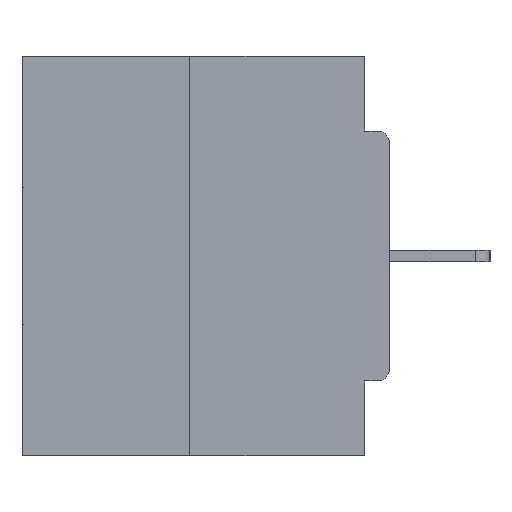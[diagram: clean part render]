
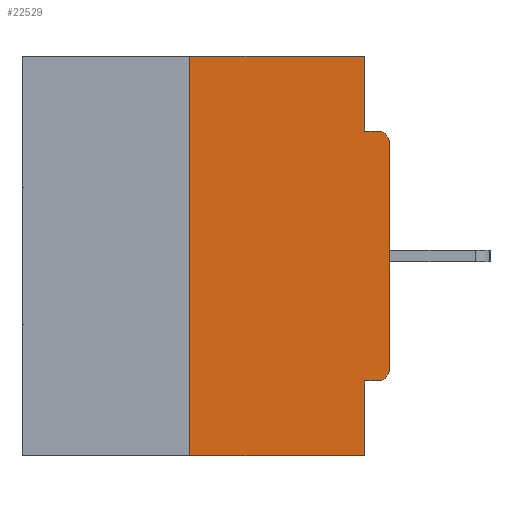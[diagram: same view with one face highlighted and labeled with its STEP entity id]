
A CAD part, left-side view. The second image highlights one B-rep face of the part: STEP entity #22529.
In plain terms, the highlighted planar face has unit normal (-1, 0, 0).
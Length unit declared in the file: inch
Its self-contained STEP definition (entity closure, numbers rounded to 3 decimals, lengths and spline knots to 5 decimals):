
#791 = VERTEX_POINT ( 'NONE', #9020 ) ;
#836 = ORIENTED_EDGE ( 'NONE', *, *, #27586, .F. ) ;
#877 = ORIENTED_EDGE ( 'NONE', *, *, #22318, .F. ) ;
#1056 = DIRECTION ( 'NONE',  ( 0., -1., 0. ) ) ;
#1707 = VECTOR ( 'NONE', #7254, 39.37008 ) ;
#1760 = CARTESIAN_POINT ( 'NONE',  ( 0., 0.25, 0. ) ) ;
#1771 = CIRCLE ( 'NONE', #20552, 0.015 ) ;
#2193 = CARTESIAN_POINT ( 'NONE',  ( 0., 0.46, 0. ) ) ;
#2301 = CARTESIAN_POINT ( 'NONE',  ( 0., 0., -0.0935 ) ) ;
#2384 = DIRECTION ( 'NONE',  ( 0., 0., -1. ) ) ;
#2485 = ORIENTED_EDGE ( 'NONE', *, *, #24553, .T. ) ;
#3978 = CARTESIAN_POINT ( 'NONE',  ( 0., 0.031, -0.4065 ) ) ;
#4126 = LINE ( 'NONE', #1760, #17793 ) ;
#4896 = LINE ( 'NONE', #2193, #1707 ) ;
#6271 = LINE ( 'NONE', #9110, #28137 ) ;
#6667 = DIRECTION ( 'NONE',  ( -1., 0., 0. ) ) ;
#6724 = ORIENTED_EDGE ( 'NONE', *, *, #23701, .F. ) ;
#7254 = DIRECTION ( 'NONE',  ( 0., -1., 0. ) ) ;
#7562 = ORIENTED_EDGE ( 'NONE', *, *, #19030, .T. ) ;
#7564 = DIRECTION ( 'NONE',  ( 0., 0., -1. ) ) ;
#7606 = CARTESIAN_POINT ( 'NONE',  ( 0., 0., -0.1085 ) ) ;
#7730 = EDGE_CURVE ( 'NONE', #12443, #24600, #21650, .T. ) ;
#8236 = DIRECTION ( 'NONE',  ( 1., 0., 0. ) ) ;
#8648 = VERTEX_POINT ( 'NONE', #8951 ) ;
#8951 = CARTESIAN_POINT ( 'NONE',  ( 0., 0.25, -0.5 ) ) ;
#9020 = CARTESIAN_POINT ( 'NONE',  ( 0., 0.25, 0. ) ) ;
#9110 = CARTESIAN_POINT ( 'NONE',  ( 0., 0.46, -0.5 ) ) ;
#9369 = VERTEX_POINT ( 'NONE', #7606 ) ;
#9497 = DIRECTION ( 'NONE',  ( 0., 1., 0. ) ) ;
#10043 = DIRECTION ( 'NONE',  ( 0., -1., 0. ) ) ;
#10325 = AXIS2_PLACEMENT_3D ( 'NONE', #11371, #6667, #31983 ) ;
#10367 = DIRECTION ( 'NONE',  ( 0., 0., -1. ) ) ;
#10672 = CARTESIAN_POINT ( 'NONE',  ( 0., 0.031, -0.5 ) ) ;
#10738 = PLANE ( 'NONE',  #13516 ) ;
#10947 = CIRCLE ( 'NONE', #10325, 0.015 ) ;
#11210 = CARTESIAN_POINT ( 'NONE',  ( 0., 0., 0. ) ) ;
#11371 = CARTESIAN_POINT ( 'NONE',  ( 0., 0.015, -0.1085 ) ) ;
#11463 = VERTEX_POINT ( 'NONE', #15191 ) ;
#12011 = CARTESIAN_POINT ( 'NONE',  ( 0., 0., -0.4065 ) ) ;
#12413 = EDGE_CURVE ( 'NONE', #12443, #31943, #1771, .T. ) ;
#12443 = VERTEX_POINT ( 'NONE', #15111 ) ;
#13076 = DIRECTION ( 'NONE',  ( -1., 0., 0. ) ) ;
#13516 = AXIS2_PLACEMENT_3D ( 'NONE', #20999, #8236, #7564 ) ;
#13811 = CARTESIAN_POINT ( 'NONE',  ( 0., 0., -0.3915 ) ) ;
#14235 = ORIENTED_EDGE ( 'NONE', *, *, #12413, .T. ) ;
#15111 = CARTESIAN_POINT ( 'NONE',  ( 0., 0.015, -0.4065 ) ) ;
#15191 = CARTESIAN_POINT ( 'NONE',  ( 0., 0.031, -0.0935 ) ) ;
#15287 = CARTESIAN_POINT ( 'NONE',  ( 0., 0.015, -0.3915 ) ) ;
#15646 = VECTOR ( 'NONE', #29152, 39.37008 ) ;
#15735 = LINE ( 'NONE', #2301, #27590 ) ;
#16244 = CARTESIAN_POINT ( 'NONE',  ( 0., 0.031, 0. ) ) ;
#17594 = VERTEX_POINT ( 'NONE', #16244 ) ;
#17793 = VECTOR ( 'NONE', #24642, 39.37008 ) ;
#18171 = FACE_OUTER_BOUND ( 'NONE', #25778, .T. ) ;
#18638 = EDGE_CURVE ( 'NONE', #8648, #791, #4126, .T. ) ;
#18850 = CARTESIAN_POINT ( 'NONE',  ( 0., 0.031, -0.5 ) ) ;
#19030 = EDGE_CURVE ( 'NONE', #31943, #9369, #29473, .T. ) ;
#20552 = AXIS2_PLACEMENT_3D ( 'NONE', #15287, #13076, #10367 ) ;
#20999 = CARTESIAN_POINT ( 'NONE',  ( 0., 0.46, 0. ) ) ;
#21650 = LINE ( 'NONE', #12011, #28503 ) ;
#22318 = EDGE_CURVE ( 'NONE', #791, #17594, #4896, .T. ) ;
#22529 = ADVANCED_FACE ( 'NONE', ( #18171 ), #10738, .F. ) ;
#23585 = CARTESIAN_POINT ( 'NONE',  ( 0., 0.015, -0.0935 ) ) ;
#23701 = EDGE_CURVE ( 'NONE', #24600, #27764, #29403, .T. ) ;
#24553 = EDGE_CURVE ( 'NONE', #9369, #30295, #10947, .T. ) ;
#24600 = VERTEX_POINT ( 'NONE', #3978 ) ;
#24642 = DIRECTION ( 'NONE',  ( 0., 0., 1. ) ) ;
#25425 = CARTESIAN_POINT ( 'NONE',  ( 0., 0.031, 0. ) ) ;
#25778 = EDGE_LOOP ( 'NONE', ( #877, #33050, #26425, #6724, #27599, #14235, #7562, #2485, #836, #31913 ) ) ;
#26425 = ORIENTED_EDGE ( 'NONE', *, *, #26475, .T. ) ;
#26475 = EDGE_CURVE ( 'NONE', #8648, #27764, #6271, .T. ) ;
#27024 = VECTOR ( 'NONE', #2384, 39.37008 ) ;
#27586 = EDGE_CURVE ( 'NONE', #11463, #30295, #15735, .T. ) ;
#27590 = VECTOR ( 'NONE', #10043, 39.37008 ) ;
#27599 = ORIENTED_EDGE ( 'NONE', *, *, #7730, .F. ) ;
#27764 = VERTEX_POINT ( 'NONE', #10672 ) ;
#27952 = EDGE_CURVE ( 'NONE', #17594, #11463, #29635, .T. ) ;
#28137 = VECTOR ( 'NONE', #1056, 39.37008 ) ;
#28503 = VECTOR ( 'NONE', #9497, 39.37008 ) ;
#28587 = VECTOR ( 'NONE', #29066, 39.37008 ) ;
#29066 = DIRECTION ( 'NONE',  ( 0., 0., -1. ) ) ;
#29152 = DIRECTION ( 'NONE',  ( 0., 0., 1. ) ) ;
#29403 = LINE ( 'NONE', #18850, #28587 ) ;
#29473 = LINE ( 'NONE', #11210, #15646 ) ;
#29635 = LINE ( 'NONE', #25425, #27024 ) ;
#30295 = VERTEX_POINT ( 'NONE', #23585 ) ;
#31913 = ORIENTED_EDGE ( 'NONE', *, *, #27952, .F. ) ;
#31943 = VERTEX_POINT ( 'NONE', #13811 ) ;
#31983 = DIRECTION ( 'NONE',  ( 0., 0., -1. ) ) ;
#33050 = ORIENTED_EDGE ( 'NONE', *, *, #18638, .F. ) ;
